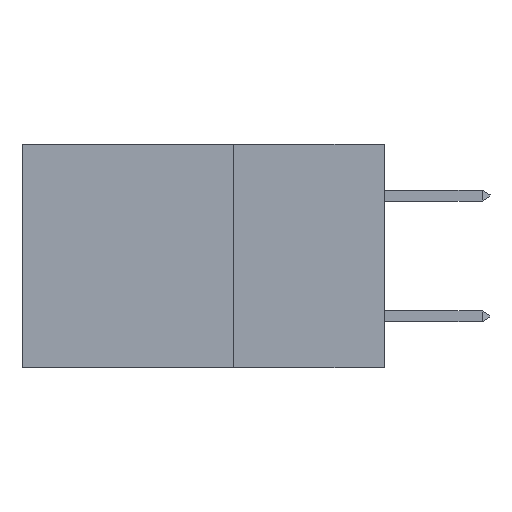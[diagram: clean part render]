
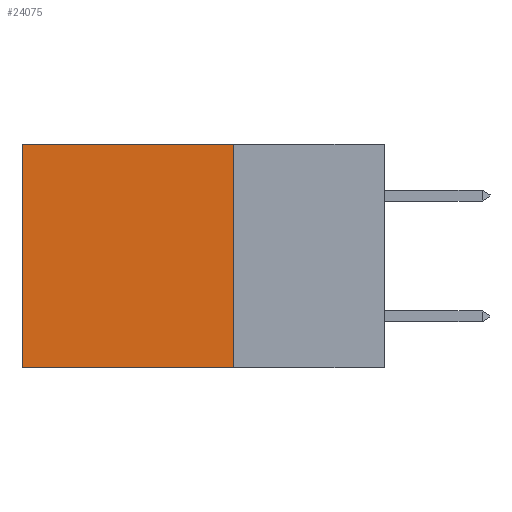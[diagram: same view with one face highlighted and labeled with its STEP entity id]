
A CAD part, left-side view. The second image highlights one B-rep face of the part: STEP entity #24075.
In plain terms, the highlighted planar face has unit normal (-1, 0, 0).
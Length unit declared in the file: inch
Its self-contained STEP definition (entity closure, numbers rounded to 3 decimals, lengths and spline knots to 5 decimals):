
#2317 = LINE ( 'NONE', #44795, #11597 ) ;
#2433 = DIRECTION ( 'NONE',  ( 0., 0., -1. ) ) ;
#7791 = PLANE ( 'NONE',  #31172 ) ;
#9344 = VECTOR ( 'NONE', #33194, 39.37008 ) ;
#11133 = DIRECTION ( 'NONE',  ( 1., 0., 0. ) ) ;
#11209 = VECTOR ( 'NONE', #19109, 39.37008 ) ;
#11597 = VECTOR ( 'NONE', #2433, 39.37008 ) ;
#11863 = EDGE_LOOP ( 'NONE', ( #38355, #29724, #30796, #37867 ) ) ;
#12435 = CARTESIAN_POINT ( 'NONE',  ( 0.2875, 0.6, -0.37 ) ) ;
#14592 = VERTEX_POINT ( 'NONE', #21667 ) ;
#14966 = CARTESIAN_POINT ( 'NONE',  ( 0.2875, 0.25, 0. ) ) ;
#18059 = VERTEX_POINT ( 'NONE', #12435 ) ;
#19109 = DIRECTION ( 'NONE',  ( 0., 1., 0. ) ) ;
#19699 = VERTEX_POINT ( 'NONE', #34028 ) ;
#21667 = CARTESIAN_POINT ( 'NONE',  ( 0.2875, 0.6, 0. ) ) ;
#23535 = VECTOR ( 'NONE', #37102, 39.37008 ) ;
#24075 = ADVANCED_FACE ( 'NONE', ( #34990 ), #7791, .F. ) ;
#28459 = CARTESIAN_POINT ( 'NONE',  ( 0.2875, 0.25, 0. ) ) ;
#29033 = LINE ( 'NONE', #33044, #9344 ) ;
#29724 = ORIENTED_EDGE ( 'NONE', *, *, #42355, .F. ) ;
#30796 = ORIENTED_EDGE ( 'NONE', *, *, #40614, .F. ) ;
#31172 = AXIS2_PLACEMENT_3D ( 'NONE', #14966, #11133, #39442 ) ;
#32499 = EDGE_CURVE ( 'NONE', #14592, #18059, #36669, .T. ) ;
#33044 = CARTESIAN_POINT ( 'NONE',  ( 0.2875, 0.25, 0. ) ) ;
#33194 = DIRECTION ( 'NONE',  ( 0., 1., 0. ) ) ;
#33632 = LINE ( 'NONE', #43732, #11209 ) ;
#34028 = CARTESIAN_POINT ( 'NONE',  ( 0.2875, 0.25, -0.37 ) ) ;
#34990 = FACE_OUTER_BOUND ( 'NONE', #11863, .T. ) ;
#35005 = VERTEX_POINT ( 'NONE', #28459 ) ;
#36669 = LINE ( 'NONE', #44019, #23535 ) ;
#37102 = DIRECTION ( 'NONE',  ( 0., 0., -1. ) ) ;
#37867 = ORIENTED_EDGE ( 'NONE', *, *, #41752, .T. ) ;
#38355 = ORIENTED_EDGE ( 'NONE', *, *, #32499, .T. ) ;
#39442 = DIRECTION ( 'NONE',  ( 0., 0., -1. ) ) ;
#40614 = EDGE_CURVE ( 'NONE', #35005, #19699, #2317, .T. ) ;
#41752 = EDGE_CURVE ( 'NONE', #35005, #14592, #29033, .T. ) ;
#42355 = EDGE_CURVE ( 'NONE', #19699, #18059, #33632, .T. ) ;
#43732 = CARTESIAN_POINT ( 'NONE',  ( 0.2875, 0.25, -0.37 ) ) ;
#44019 = CARTESIAN_POINT ( 'NONE',  ( 0.2875, 0.6, 0. ) ) ;
#44795 = CARTESIAN_POINT ( 'NONE',  ( 0.2875, 0.25, 0. ) ) ;
